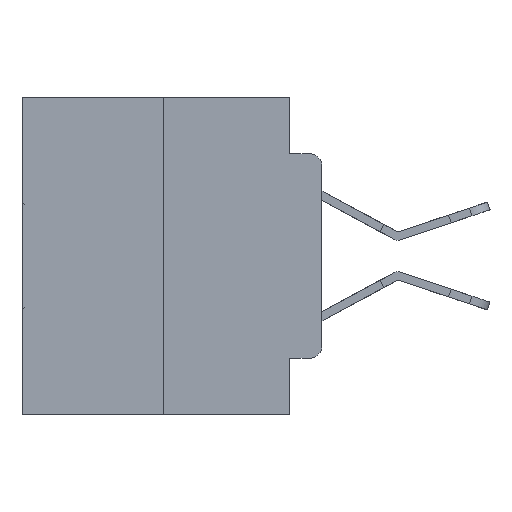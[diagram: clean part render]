
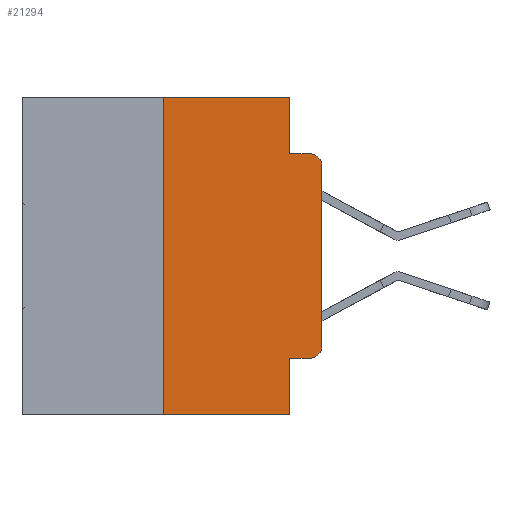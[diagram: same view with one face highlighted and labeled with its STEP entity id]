
A CAD part, left-side view. The second image highlights one B-rep face of the part: STEP entity #21294.
In plain terms, the highlighted planar face has unit normal (-1, 0, 0).
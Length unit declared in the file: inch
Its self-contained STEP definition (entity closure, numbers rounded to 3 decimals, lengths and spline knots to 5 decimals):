
#47 = VECTOR ( 'NONE', #28782, 39.37008 ) ;
#221 = VERTEX_POINT ( 'NONE', #6956 ) ;
#640 = LINE ( 'NONE', #8929, #12309 ) ;
#1835 = CARTESIAN_POINT ( 'NONE',  ( 0., 0.02, -0.1085 ) ) ;
#1905 = EDGE_CURVE ( 'NONE', #221, #11817, #640, .T. ) ;
#2114 = DIRECTION ( 'NONE',  ( 0., -1., 0. ) ) ;
#2408 = EDGE_CURVE ( 'NONE', #11940, #28905, #29027, .T. ) ;
#2953 = VERTEX_POINT ( 'NONE', #9615 ) ;
#2999 = ORIENTED_EDGE ( 'NONE', *, *, #3923, .F. ) ;
#3165 = EDGE_CURVE ( 'NONE', #2953, #11460, #28350, .T. ) ;
#3594 = LINE ( 'NONE', #27983, #27246 ) ;
#3874 = CARTESIAN_POINT ( 'NONE',  ( 0., 0.473, 0. ) ) ;
#3923 = EDGE_CURVE ( 'NONE', #24988, #11460, #3594, .T. ) ;
#4224 = DIRECTION ( 'NONE',  ( 0., 0., -1. ) ) ;
#4396 = CARTESIAN_POINT ( 'NONE',  ( 0., 0.25, 0. ) ) ;
#5481 = EDGE_CURVE ( 'NONE', #24988, #11940, #24629, .T. ) ;
#5512 = DIRECTION ( 'NONE',  ( 0., -1., 0. ) ) ;
#5702 = VERTEX_POINT ( 'NONE', #11735 ) ;
#6236 = DIRECTION ( 'NONE',  ( 0., 0., 1. ) ) ;
#6258 = ORIENTED_EDGE ( 'NONE', *, *, #14528, .F. ) ;
#6333 = LINE ( 'NONE', #29536, #11729 ) ;
#6807 = CARTESIAN_POINT ( 'NONE',  ( 0., 0., -0.1085 ) ) ;
#6956 = CARTESIAN_POINT ( 'NONE',  ( 0., 0.051, 0. ) ) ;
#7106 = VECTOR ( 'NONE', #22348, 39.37008 ) ;
#7859 = LINE ( 'NONE', #24547, #7106 ) ;
#7893 = CARTESIAN_POINT ( 'NONE',  ( 0., 0., -0.3915 ) ) ;
#8462 = ORIENTED_EDGE ( 'NONE', *, *, #20612, .F. ) ;
#8536 = DIRECTION ( 'NONE',  ( 0., 0., -1. ) ) ;
#8804 = ORIENTED_EDGE ( 'NONE', *, *, #12850, .T. ) ;
#8929 = CARTESIAN_POINT ( 'NONE',  ( 0., 0.051, 0. ) ) ;
#9342 = DIRECTION ( 'NONE',  ( -1., 0., 0. ) ) ;
#9615 = CARTESIAN_POINT ( 'NONE',  ( 0., 0.25, -0.5 ) ) ;
#9882 = ORIENTED_EDGE ( 'NONE', *, *, #5481, .T. ) ;
#10142 = VECTOR ( 'NONE', #11017, 39.37008 ) ;
#10598 = ORIENTED_EDGE ( 'NONE', *, *, #2408, .T. ) ;
#10627 = LINE ( 'NONE', #12450, #17417 ) ;
#10942 = ORIENTED_EDGE ( 'NONE', *, *, #1905, .F. ) ;
#11017 = DIRECTION ( 'NONE',  ( 0., -1., 0. ) ) ;
#11460 = VERTEX_POINT ( 'NONE', #28786 ) ;
#11624 = AXIS2_PLACEMENT_3D ( 'NONE', #1835, #17965, #4224 ) ;
#11729 = VECTOR ( 'NONE', #2114, 39.37008 ) ;
#11735 = CARTESIAN_POINT ( 'NONE',  ( 0., 0.02, -0.0885 ) ) ;
#11817 = VERTEX_POINT ( 'NONE', #14030 ) ;
#11940 = VERTEX_POINT ( 'NONE', #12225 ) ;
#12225 = CARTESIAN_POINT ( 'NONE',  ( 0., 0.02, -0.4115 ) ) ;
#12309 = VECTOR ( 'NONE', #20128, 39.37008 ) ;
#12411 = FACE_OUTER_BOUND ( 'NONE', #19036, .T. ) ;
#12450 = CARTESIAN_POINT ( 'NONE',  ( 0., 0.051, -0.0885 ) ) ;
#12507 = AXIS2_PLACEMENT_3D ( 'NONE', #16775, #9342, #8536 ) ;
#12766 = DIRECTION ( 'NONE',  ( 0., 0., -1. ) ) ;
#12850 = EDGE_CURVE ( 'NONE', #28905, #19637, #7859, .T. ) ;
#13141 = DIRECTION ( 'NONE',  ( 0., 0., -1. ) ) ;
#14030 = CARTESIAN_POINT ( 'NONE',  ( 0., 0.051, -0.0885 ) ) ;
#14528 = EDGE_CURVE ( 'NONE', #26364, #221, #6333, .T. ) ;
#14541 = ORIENTED_EDGE ( 'NONE', *, *, #3165, .T. ) ;
#14967 = VECTOR ( 'NONE', #6236, 39.37008 ) ;
#15150 = CARTESIAN_POINT ( 'NONE',  ( 0., 0.051, -0.4115 ) ) ;
#16775 = CARTESIAN_POINT ( 'NONE',  ( 0., 0.02, -0.3915 ) ) ;
#17417 = VECTOR ( 'NONE', #5512, 39.37008 ) ;
#17629 = PLANE ( 'NONE',  #29628 ) ;
#17965 = DIRECTION ( 'NONE',  ( -1., 0., 0. ) ) ;
#19036 = EDGE_LOOP ( 'NONE', ( #8804, #27013, #28425, #10942, #6258, #8462, #14541, #2999, #9882, #10598 ) ) ;
#19636 = LINE ( 'NONE', #19985, #14967 ) ;
#19637 = VERTEX_POINT ( 'NONE', #6807 ) ;
#19985 = CARTESIAN_POINT ( 'NONE',  ( 0., 0.25, 0. ) ) ;
#20128 = DIRECTION ( 'NONE',  ( 0., 0., -1. ) ) ;
#20612 = EDGE_CURVE ( 'NONE', #2953, #26364, #19636, .T. ) ;
#21294 = ADVANCED_FACE ( 'NONE', ( #12411 ), #17629, .F. ) ;
#22348 = DIRECTION ( 'NONE',  ( 0., 0., 1. ) ) ;
#24547 = CARTESIAN_POINT ( 'NONE',  ( 0., 0., 0. ) ) ;
#24629 = LINE ( 'NONE', #15150, #47 ) ;
#24988 = VERTEX_POINT ( 'NONE', #27886 ) ;
#26011 = EDGE_CURVE ( 'NONE', #11817, #5702, #10627, .T. ) ;
#26364 = VERTEX_POINT ( 'NONE', #4396 ) ;
#26810 = DIRECTION ( 'NONE',  ( 1., 0., 0. ) ) ;
#27013 = ORIENTED_EDGE ( 'NONE', *, *, #27532, .T. ) ;
#27246 = VECTOR ( 'NONE', #12766, 39.37008 ) ;
#27532 = EDGE_CURVE ( 'NONE', #19637, #5702, #28377, .T. ) ;
#27886 = CARTESIAN_POINT ( 'NONE',  ( 0., 0.051, -0.4115 ) ) ;
#27983 = CARTESIAN_POINT ( 'NONE',  ( 0., 0.051, 0. ) ) ;
#28350 = LINE ( 'NONE', #29375, #10142 ) ;
#28377 = CIRCLE ( 'NONE', #11624, 0.02 ) ;
#28425 = ORIENTED_EDGE ( 'NONE', *, *, #26011, .F. ) ;
#28782 = DIRECTION ( 'NONE',  ( 0., -1., 0. ) ) ;
#28786 = CARTESIAN_POINT ( 'NONE',  ( 0., 0.051, -0.5 ) ) ;
#28905 = VERTEX_POINT ( 'NONE', #7893 ) ;
#29027 = CIRCLE ( 'NONE', #12507, 0.02 ) ;
#29375 = CARTESIAN_POINT ( 'NONE',  ( 0., 0.473, -0.5 ) ) ;
#29536 = CARTESIAN_POINT ( 'NONE',  ( 0., 0.473, 0. ) ) ;
#29628 = AXIS2_PLACEMENT_3D ( 'NONE', #3874, #26810, #13141 ) ;
